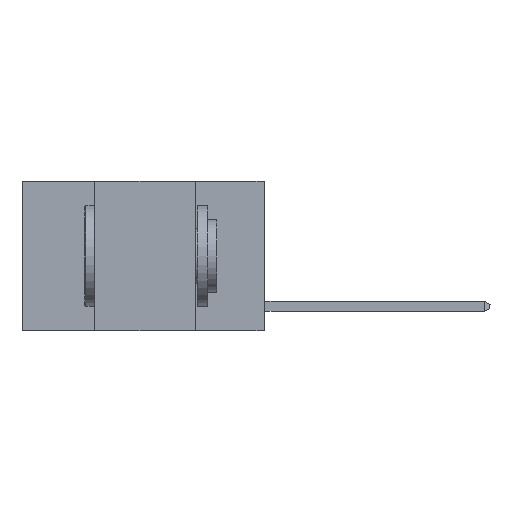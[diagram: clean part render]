
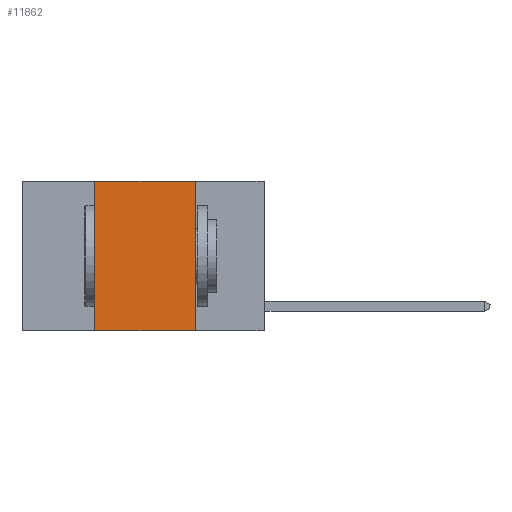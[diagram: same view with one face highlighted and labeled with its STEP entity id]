
A CAD part, left-side view. The second image highlights one B-rep face of the part: STEP entity #11862.
In plain terms, the highlighted planar face has unit normal (-1, 0, 0).
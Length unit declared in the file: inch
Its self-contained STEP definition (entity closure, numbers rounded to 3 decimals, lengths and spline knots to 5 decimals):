
#268 = DIRECTION ( 'NONE',  ( 0., -1., 0. ) ) ;
#523 = ORIENTED_EDGE ( 'NONE', *, *, #14350, .T. ) ;
#1300 = EDGE_CURVE ( 'NONE', #19870, #5998, #3854, .T. ) ;
#1904 = DIRECTION ( 'NONE',  ( 0., 0., 1. ) ) ;
#2422 = ORIENTED_EDGE ( 'NONE', *, *, #19106, .F. ) ;
#3854 = LINE ( 'NONE', #17919, #11761 ) ;
#5312 = ORIENTED_EDGE ( 'NONE', *, *, #1300, .F. ) ;
#5479 = EDGE_CURVE ( 'NONE', #5998, #20507, #23253, .T. ) ;
#5974 = CARTESIAN_POINT ( 'NONE',  ( 0., 0.17, 0. ) ) ;
#5998 = VERTEX_POINT ( 'NONE', #16722 ) ;
#6380 = CARTESIAN_POINT ( 'NONE',  ( 0., 0.6, 0. ) ) ;
#6612 = VERTEX_POINT ( 'NONE', #18233 ) ;
#7419 = CARTESIAN_POINT ( 'NONE',  ( 0., 0.6, -0.37 ) ) ;
#8275 = CARTESIAN_POINT ( 'NONE',  ( 0., 0.42, -0.37 ) ) ;
#8731 = VECTOR ( 'NONE', #16981, 39.37008 ) ;
#10191 = FACE_OUTER_BOUND ( 'NONE', #17707, .T. ) ;
#11761 = VECTOR ( 'NONE', #1904, 39.37008 ) ;
#11833 = CARTESIAN_POINT ( 'NONE',  ( 0., 0.6, 0. ) ) ;
#11862 = ADVANCED_FACE ( 'NONE', ( #10191 ), #13762, .F. ) ;
#13046 = DIRECTION ( 'NONE',  ( 0., 0., -1. ) ) ;
#13078 = AXIS2_PLACEMENT_3D ( 'NONE', #6380, #22907, #19069 ) ;
#13762 = PLANE ( 'NONE',  #13078 ) ;
#14285 = ORIENTED_EDGE ( 'NONE', *, *, #5479, .F. ) ;
#14350 = EDGE_CURVE ( 'NONE', #19870, #6612, #23364, .T. ) ;
#16244 = VECTOR ( 'NONE', #13046, 39.37008 ) ;
#16722 = CARTESIAN_POINT ( 'NONE',  ( 0., 0.42, 0. ) ) ;
#16981 = DIRECTION ( 'NONE',  ( 0., -1., 0. ) ) ;
#17707 = EDGE_LOOP ( 'NONE', ( #2422, #14285, #5312, #523 ) ) ;
#17919 = CARTESIAN_POINT ( 'NONE',  ( 0., 0.42, 0. ) ) ;
#18233 = CARTESIAN_POINT ( 'NONE',  ( 0., 0.17, -0.37 ) ) ;
#18498 = VECTOR ( 'NONE', #268, 39.37008 ) ;
#19069 = DIRECTION ( 'NONE',  ( 0., 0., -1. ) ) ;
#19106 = EDGE_CURVE ( 'NONE', #20507, #6612, #19963, .T. ) ;
#19870 = VERTEX_POINT ( 'NONE', #8275 ) ;
#19963 = LINE ( 'NONE', #5974, #16244 ) ;
#20507 = VERTEX_POINT ( 'NONE', #21194 ) ;
#21194 = CARTESIAN_POINT ( 'NONE',  ( 0., 0.17, 0. ) ) ;
#22907 = DIRECTION ( 'NONE',  ( 1., 0., 0. ) ) ;
#23253 = LINE ( 'NONE', #11833, #8731 ) ;
#23364 = LINE ( 'NONE', #7419, #18498 ) ;
